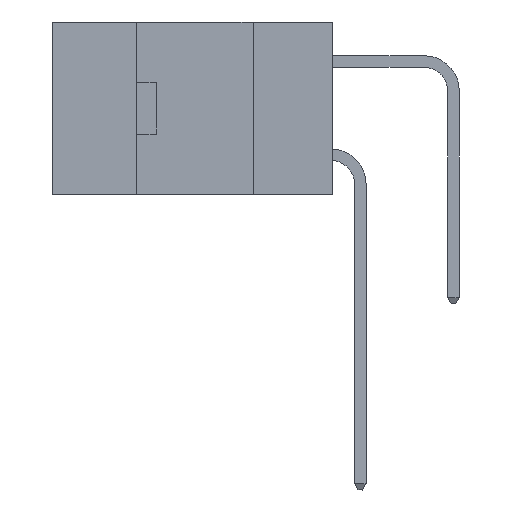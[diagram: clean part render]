
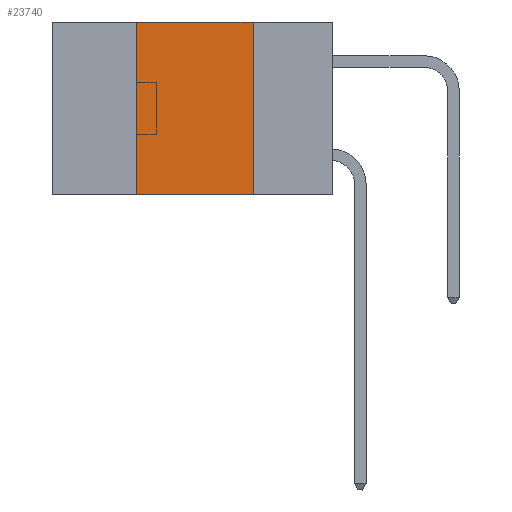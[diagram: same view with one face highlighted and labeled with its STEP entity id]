
A CAD part, left-side view. The second image highlights one B-rep face of the part: STEP entity #23740.
In plain terms, the highlighted planar face has unit normal (-1, 0, 0).
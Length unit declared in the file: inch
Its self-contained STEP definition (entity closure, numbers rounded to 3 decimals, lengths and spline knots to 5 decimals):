
#627 = DIRECTION ( 'NONE',  ( 0., 0., 1. ) ) ;
#1440 = ORIENTED_EDGE ( 'NONE', *, *, #18167, .T. ) ;
#1496 = VECTOR ( 'NONE', #24881, 39.37008 ) ;
#2092 = VERTEX_POINT ( 'NONE', #18487 ) ;
#2691 = LINE ( 'NONE', #26602, #8272 ) ;
#3522 = EDGE_CURVE ( 'NONE', #2092, #8893, #12171, .T. ) ;
#4926 = DIRECTION ( 'NONE',  ( 0., 0., -1. ) ) ;
#6904 = VERTEX_POINT ( 'NONE', #11002 ) ;
#7048 = DIRECTION ( 'NONE',  ( 0., -1., 0. ) ) ;
#7282 = CARTESIAN_POINT ( 'NONE',  ( 0., 0.42, -0.37 ) ) ;
#7654 = CARTESIAN_POINT ( 'NONE',  ( 0., 0.6, 0. ) ) ;
#7794 = VECTOR ( 'NONE', #7048, 39.37008 ) ;
#8088 = EDGE_CURVE ( 'NONE', #29839, #2092, #29214, .T. ) ;
#8109 = AXIS2_PLACEMENT_3D ( 'NONE', #19058, #16711, #4926 ) ;
#8272 = VECTOR ( 'NONE', #12155, 39.37008 ) ;
#8893 = VERTEX_POINT ( 'NONE', #14657 ) ;
#11002 = CARTESIAN_POINT ( 'NONE',  ( 0., 0.17, -0.37 ) ) ;
#12062 = VECTOR ( 'NONE', #627, 39.37008 ) ;
#12155 = DIRECTION ( 'NONE',  ( 0., 0., -1. ) ) ;
#12171 = LINE ( 'NONE', #7654, #7794 ) ;
#12369 = EDGE_CURVE ( 'NONE', #8893, #6904, #2691, .T. ) ;
#14657 = CARTESIAN_POINT ( 'NONE',  ( 0., 0.17, 0. ) ) ;
#16711 = DIRECTION ( 'NONE',  ( 1., 0., 0. ) ) ;
#17224 = CARTESIAN_POINT ( 'NONE',  ( 0., 0.42, -0.37 ) ) ;
#17724 = LINE ( 'NONE', #29872, #1496 ) ;
#18167 = EDGE_CURVE ( 'NONE', #29839, #6904, #17724, .T. ) ;
#18487 = CARTESIAN_POINT ( 'NONE',  ( 0., 0.42, 0. ) ) ;
#18660 = ORIENTED_EDGE ( 'NONE', *, *, #3522, .F. ) ;
#19058 = CARTESIAN_POINT ( 'NONE',  ( 0., 0.6, 0. ) ) ;
#21161 = ORIENTED_EDGE ( 'NONE', *, *, #8088, .F. ) ;
#23740 = ADVANCED_FACE ( 'NONE', ( #25754 ), #26214, .F. ) ;
#24037 = ORIENTED_EDGE ( 'NONE', *, *, #12369, .F. ) ;
#24881 = DIRECTION ( 'NONE',  ( 0., -1., 0. ) ) ;
#25754 = FACE_OUTER_BOUND ( 'NONE', #26069, .T. ) ;
#26069 = EDGE_LOOP ( 'NONE', ( #24037, #18660, #21161, #1440 ) ) ;
#26214 = PLANE ( 'NONE',  #8109 ) ;
#26602 = CARTESIAN_POINT ( 'NONE',  ( 0., 0.17, -0.37 ) ) ;
#29214 = LINE ( 'NONE', #17224, #12062 ) ;
#29839 = VERTEX_POINT ( 'NONE', #7282 ) ;
#29872 = CARTESIAN_POINT ( 'NONE',  ( 0., 0.6, -0.37 ) ) ;
